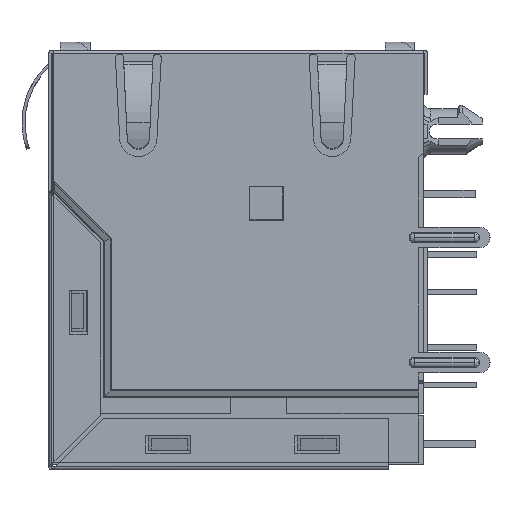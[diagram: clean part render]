
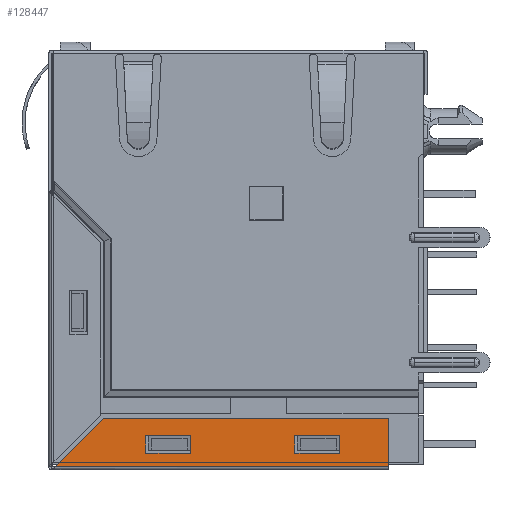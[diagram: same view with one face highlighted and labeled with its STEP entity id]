
A CAD part, left-side view. The second image highlights one B-rep face of the part: STEP entity #128447.
In plain terms, the highlighted planar face has unit normal (-1, 0, 0).
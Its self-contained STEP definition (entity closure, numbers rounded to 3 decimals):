
#3830 = AXIS2_PLACEMENT_3D ( 'NONE', #78182, #8803, #136327 ) ;
#5821 = B_SPLINE_CURVE_WITH_KNOTS ( 'NONE', 1,
 ( #99773, #8613 ),
 .UNSPECIFIED., .F., .F.,
 ( 2, 2 ),
 ( 0., 1. ),
 .UNSPECIFIED. ) ;
#6752 = ORIENTED_EDGE ( 'NONE', *, *, #29801, .F. ) ;
#8613 = CARTESIAN_POINT ( 'NONE',  ( -31.875, 6.165, -26.78 ) ) ;
#8635 = ORIENTED_EDGE ( 'NONE', *, *, #68755, .F. ) ;
#8803 = DIRECTION ( 'NONE',  ( -1., 0., 0. ) ) ;
#10635 = B_SPLINE_CURVE_WITH_KNOTS ( 'NONE', 1,
 ( #23439, #13783 ),
 .UNSPECIFIED., .F., .F.,
 ( 2, 2 ),
 ( 0., 1. ),
 .UNSPECIFIED. ) ;
#11320 = ORIENTED_EDGE ( 'NONE', *, *, #126916, .T. ) ;
#13783 = CARTESIAN_POINT ( 'NONE',  ( -31.875, -6.835, -26.78 ) ) ;
#14411 = EDGE_LOOP ( 'NONE', ( #79707, #101958, #11320, #89522 ) ) ;
#17528 = CARTESIAN_POINT ( 'NONE',  ( -31.875, 6.165, -25.58 ) ) ;
#18120 = CARTESIAN_POINT ( 'NONE',  ( -31.875, -3.835, -26.78 ) ) ;
#19685 = CARTESIAN_POINT ( 'NONE',  ( -31.875, 3.165, -25.58 ) ) ;
#20835 = EDGE_CURVE ( 'NONE', #126411, #113634, #58455, .T. ) ;
#23439 = CARTESIAN_POINT ( 'NONE',  ( -31.875, -6.835, -25.58 ) ) ;
#24551 = EDGE_CURVE ( 'NONE', #146261, #62431, #111211, .T. ) ;
#25834 = FACE_BOUND ( 'NONE', #57985, .T. ) ;
#27672 = CARTESIAN_POINT ( 'NONE',  ( -31.875, -3.835, -26.78 ) ) ;
#29141 = ORIENTED_EDGE ( 'NONE', *, *, #91120, .T. ) ;
#29486 = B_SPLINE_CURVE_WITH_KNOTS ( 'NONE', 1,
 ( #38756, #84339 ),
 .UNSPECIFIED., .F., .F.,
 ( 2, 2 ),
 ( 0., 1. ),
 .UNSPECIFIED. ) ;
#29801 = EDGE_CURVE ( 'NONE', #43678, #50803, #122323, .T. ) ;
#31042 = B_SPLINE_CURVE_WITH_KNOTS ( 'NONE', 1,
 ( #84119, #139777 ),
 .UNSPECIFIED., .F., .F.,
 ( 2, 2 ),
 ( 0., 1. ),
 .UNSPECIFIED. ) ;
#31665 = CARTESIAN_POINT ( 'NONE',  ( -31.875, -6.835, -25.58 ) ) ;
#34604 = VERTEX_POINT ( 'NONE', #125162 ) ;
#37806 = CARTESIAN_POINT ( 'NONE',  ( -31.875, 3.165, -25.58 ) ) ;
#38756 = CARTESIAN_POINT ( 'NONE',  ( -31.875, 9.005, -24.43 ) ) ;
#39018 = EDGE_CURVE ( 'NONE', #62431, #145603, #43359, .T. ) ;
#41137 = EDGE_CURVE ( 'NONE', #34604, #50803, #116689, .T. ) ;
#41346 = EDGE_CURVE ( 'NONE', #115963, #43678, #29486, .T. ) ;
#43359 = B_SPLINE_CURVE_WITH_KNOTS ( 'NONE', 1,
 ( #18120, #52538 ),
 .UNSPECIFIED., .F., .F.,
 ( 2, 2 ),
 ( 0., 1. ),
 .UNSPECIFIED. ) ;
#43678 = VERTEX_POINT ( 'NONE', #113007 ) ;
#45813 = CARTESIAN_POINT ( 'NONE',  ( -31.875, -10.135, -24.43 ) ) ;
#50803 = VERTEX_POINT ( 'NONE', #115738 ) ;
#52538 = CARTESIAN_POINT ( 'NONE',  ( -31.875, -3.835, -25.58 ) ) ;
#57985 = EDGE_LOOP ( 'NONE', ( #103689, #60552, #29141, #135266 ) ) ;
#58455 = B_SPLINE_CURVE_WITH_KNOTS ( 'NONE', 1,
 ( #74217, #17528 ),
 .UNSPECIFIED., .F., .F.,
 ( 2, 2 ),
 ( 0., 1. ),
 .UNSPECIFIED. ) ;
#59964 = CARTESIAN_POINT ( 'NONE',  ( -31.875, -3.835, -26.78 ) ) ;
#60552 = ORIENTED_EDGE ( 'NONE', *, *, #129298, .T. ) ;
#62078 = CARTESIAN_POINT ( 'NONE',  ( -31.875, 6.165, -26.78 ) ) ;
#62431 = VERTEX_POINT ( 'NONE', #59964 ) ;
#67497 = CARTESIAN_POINT ( 'NONE',  ( -31.875, 3.165, -26.78 ) ) ;
#68475 = CARTESIAN_POINT ( 'NONE',  ( -31.875, 12.245, -27.67 ) ) ;
#68755 = EDGE_CURVE ( 'NONE', #34604, #115963, #115481, .T. ) ;
#73751 = ORIENTED_EDGE ( 'NONE', *, *, #41137, .T. ) ;
#74217 = CARTESIAN_POINT ( 'NONE',  ( -31.875, 6.165, -26.78 ) ) ;
#78182 = CARTESIAN_POINT ( 'NONE',  ( -31.875, 12.693, -27.766 ) ) ;
#78374 = B_SPLINE_CURVE_WITH_KNOTS ( 'NONE', 1,
 ( #101653, #19685 ),
 .UNSPECIFIED., .F., .F.,
 ( 2, 2 ),
 ( 0., 1. ),
 .UNSPECIFIED. ) ;
#79081 = VERTEX_POINT ( 'NONE', #67497 ) ;
#79707 = ORIENTED_EDGE ( 'NONE', *, *, #39018, .T. ) ;
#81165 = ORIENTED_EDGE ( 'NONE', *, *, #41346, .F. ) ;
#82672 = EDGE_CURVE ( 'NONE', #145603, #97368, #31042, .T. ) ;
#83804 = FACE_BOUND ( 'NONE', #14411, .T. ) ;
#84119 = CARTESIAN_POINT ( 'NONE',  ( -31.875, -3.835, -25.58 ) ) ;
#84339 = CARTESIAN_POINT ( 'NONE',  ( -31.875, -10.135, -24.43 ) ) ;
#87259 = FACE_OUTER_BOUND ( 'NONE', #104325, .T. ) ;
#89522 = ORIENTED_EDGE ( 'NONE', *, *, #24551, .T. ) ;
#89690 = B_SPLINE_CURVE_WITH_KNOTS ( 'NONE', 1,
 ( #37806, #118712 ),
 .UNSPECIFIED., .F., .F.,
 ( 2, 2 ),
 ( 0., 1. ),
 .UNSPECIFIED. ) ;
#91120 = EDGE_CURVE ( 'NONE', #115823, #79081, #89690, .T. ) ;
#91256 = CARTESIAN_POINT ( 'NONE',  ( -31.875, 9.005, -24.43 ) ) ;
#94011 = CARTESIAN_POINT ( 'NONE',  ( -31.875, 3.165, -25.58 ) ) ;
#97368 = VERTEX_POINT ( 'NONE', #31665 ) ;
#99773 = CARTESIAN_POINT ( 'NONE',  ( -31.875, 3.165, -26.78 ) ) ;
#101653 = CARTESIAN_POINT ( 'NONE',  ( -31.875, 6.165, -25.58 ) ) ;
#101958 = ORIENTED_EDGE ( 'NONE', *, *, #82672, .T. ) ;
#103689 = ORIENTED_EDGE ( 'NONE', *, *, #20835, .T. ) ;
#104325 = EDGE_LOOP ( 'NONE', ( #8635, #73751, #6752, #81165 ) ) ;
#111211 = B_SPLINE_CURVE_WITH_KNOTS ( 'NONE', 1,
 ( #142521, #27672 ),
 .UNSPECIFIED., .F., .F.,
 ( 2, 2 ),
 ( 0., 1. ),
 .UNSPECIFIED. ) ;
#113007 = CARTESIAN_POINT ( 'NONE',  ( -31.875, -10.135, -24.43 ) ) ;
#113634 = VERTEX_POINT ( 'NONE', #129462 ) ;
#114261 = CARTESIAN_POINT ( 'NONE',  ( -31.875, -3.835, -25.58 ) ) ;
#115481 = B_SPLINE_CURVE_WITH_KNOTS ( 'NONE', 1,
 ( #68475, #91256 ),
 .UNSPECIFIED., .F., .F.,
 ( 2, 2 ),
 ( 0., 1. ),
 .UNSPECIFIED. ) ;
#115738 = CARTESIAN_POINT ( 'NONE',  ( -31.875, -10.135, -27.67 ) ) ;
#115823 = VERTEX_POINT ( 'NONE', #94011 ) ;
#115963 = VERTEX_POINT ( 'NONE', #144078 ) ;
#116689 = B_SPLINE_CURVE_WITH_KNOTS ( 'NONE', 1,
 ( #138949, #125824 ),
 .UNSPECIFIED., .F., .F.,
 ( 2, 2 ),
 ( 0., 1. ),
 .UNSPECIFIED. ) ;
#118712 = CARTESIAN_POINT ( 'NONE',  ( -31.875, 3.165, -26.78 ) ) ;
#122323 = B_SPLINE_CURVE_WITH_KNOTS ( 'NONE', 1,
 ( #45813, #126253 ),
 .UNSPECIFIED., .F., .F.,
 ( 2, 2 ),
 ( 0., 1. ),
 .UNSPECIFIED. ) ;
#125162 = CARTESIAN_POINT ( 'NONE',  ( -31.875, 12.245, -27.67 ) ) ;
#125687 = PLANE ( 'NONE',  #3830 ) ;
#125824 = CARTESIAN_POINT ( 'NONE',  ( -31.875, -10.135, -27.67 ) ) ;
#126253 = CARTESIAN_POINT ( 'NONE',  ( -31.875, -10.135, -27.67 ) ) ;
#126411 = VERTEX_POINT ( 'NONE', #62078 ) ;
#126916 = EDGE_CURVE ( 'NONE', #97368, #146261, #10635, .T. ) ;
#128447 = ADVANCED_FACE ( 'NONE', ( #87259, #25834, #83804 ), #125687, .T. ) ;
#129298 = EDGE_CURVE ( 'NONE', #113634, #115823, #78374, .T. ) ;
#129462 = CARTESIAN_POINT ( 'NONE',  ( -31.875, 6.165, -25.58 ) ) ;
#135266 = ORIENTED_EDGE ( 'NONE', *, *, #144229, .T. ) ;
#136327 = DIRECTION ( 'NONE',  ( 0., -1., 0. ) ) ;
#138949 = CARTESIAN_POINT ( 'NONE',  ( -31.875, 12.245, -27.67 ) ) ;
#139777 = CARTESIAN_POINT ( 'NONE',  ( -31.875, -6.835, -25.58 ) ) ;
#142521 = CARTESIAN_POINT ( 'NONE',  ( -31.875, -6.835, -26.78 ) ) ;
#144078 = CARTESIAN_POINT ( 'NONE',  ( -31.875, 9.005, -24.43 ) ) ;
#144229 = EDGE_CURVE ( 'NONE', #79081, #126411, #5821, .T. ) ;
#144320 = CARTESIAN_POINT ( 'NONE',  ( -31.875, -6.835, -26.78 ) ) ;
#145603 = VERTEX_POINT ( 'NONE', #114261 ) ;
#146261 = VERTEX_POINT ( 'NONE', #144320 ) ;
